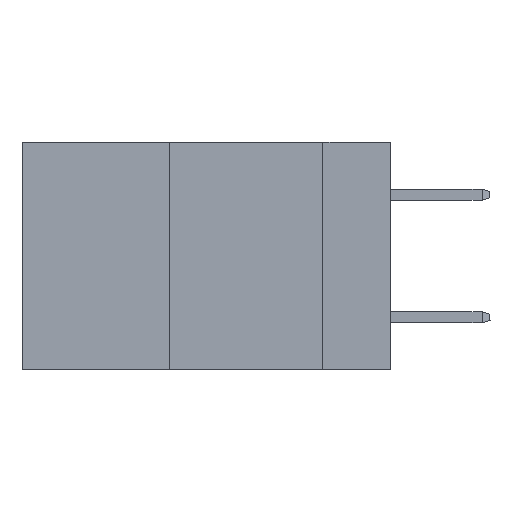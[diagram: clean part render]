
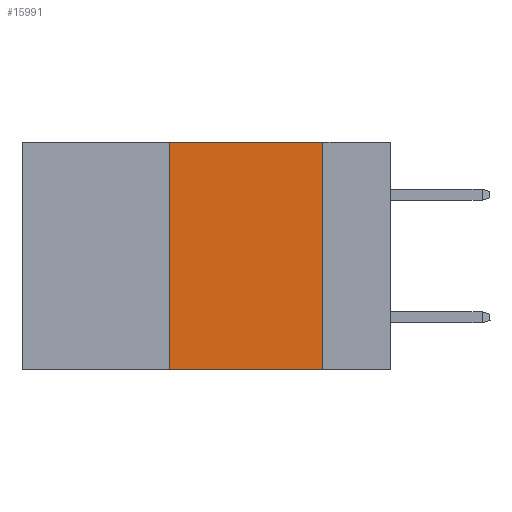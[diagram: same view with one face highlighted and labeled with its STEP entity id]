
A CAD part, left-side view. The second image highlights one B-rep face of the part: STEP entity #15991.
In plain terms, the highlighted planar face has unit normal (-1, 0, 0).
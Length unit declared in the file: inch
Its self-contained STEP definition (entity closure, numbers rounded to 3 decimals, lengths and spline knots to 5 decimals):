
#643 = CARTESIAN_POINT ( 'NONE',  ( 0., 0.6, 0. ) ) ;
#4581 = VERTEX_POINT ( 'NONE', #21005 ) ;
#7000 = EDGE_CURVE ( 'NONE', #4581, #27219, #23626, .T. ) ;
#7604 = EDGE_CURVE ( 'NONE', #27219, #26517, #26602, .T. ) ;
#8056 = AXIS2_PLACEMENT_3D ( 'NONE', #12848, #10440, #13199 ) ;
#8575 = DIRECTION ( 'NONE',  ( 0., 0., -1. ) ) ;
#10440 = DIRECTION ( 'NONE',  ( 1., 0., 0. ) ) ;
#10916 = CARTESIAN_POINT ( 'NONE',  ( 0., 0.6, -0.37 ) ) ;
#11458 = DIRECTION ( 'NONE',  ( 0., -1., 0. ) ) ;
#11513 = EDGE_LOOP ( 'NONE', ( #23986, #29584, #23904, #30124 ) ) ;
#12848 = CARTESIAN_POINT ( 'NONE',  ( 0., 0.6, 0. ) ) ;
#13199 = DIRECTION ( 'NONE',  ( 0., 0., -1. ) ) ;
#15375 = EDGE_CURVE ( 'NONE', #35137, #4581, #23863, .T. ) ;
#15991 = ADVANCED_FACE ( 'NONE', ( #25565 ), #26782, .F. ) ;
#16238 = VECTOR ( 'NONE', #19378, 39.37008 ) ;
#17116 = VECTOR ( 'NONE', #11458, 39.37008 ) ;
#19378 = DIRECTION ( 'NONE',  ( 0., -1., 0. ) ) ;
#20238 = CARTESIAN_POINT ( 'NONE',  ( 0., 0.11, -0.37 ) ) ;
#21005 = CARTESIAN_POINT ( 'NONE',  ( 0., 0.36, 0. ) ) ;
#21070 = CARTESIAN_POINT ( 'NONE',  ( 0., 0.36, 0. ) ) ;
#22234 = EDGE_CURVE ( 'NONE', #35137, #26517, #23641, .T. ) ;
#22790 = CARTESIAN_POINT ( 'NONE',  ( 0., 0.36, -0.37 ) ) ;
#23626 = LINE ( 'NONE', #643, #17116 ) ;
#23641 = LINE ( 'NONE', #10916, #16238 ) ;
#23858 = DIRECTION ( 'NONE',  ( 0., 0., 1. ) ) ;
#23863 = LINE ( 'NONE', #21070, #35088 ) ;
#23904 = ORIENTED_EDGE ( 'NONE', *, *, #15375, .F. ) ;
#23986 = ORIENTED_EDGE ( 'NONE', *, *, #7604, .F. ) ;
#24905 = CARTESIAN_POINT ( 'NONE',  ( 0., 0.11, 0. ) ) ;
#25565 = FACE_OUTER_BOUND ( 'NONE', #11513, .T. ) ;
#25589 = CARTESIAN_POINT ( 'NONE',  ( 0., 0.11, 0. ) ) ;
#26517 = VERTEX_POINT ( 'NONE', #20238 ) ;
#26602 = LINE ( 'NONE', #24905, #27023 ) ;
#26782 = PLANE ( 'NONE',  #8056 ) ;
#27023 = VECTOR ( 'NONE', #8575, 39.37008 ) ;
#27219 = VERTEX_POINT ( 'NONE', #25589 ) ;
#29584 = ORIENTED_EDGE ( 'NONE', *, *, #7000, .F. ) ;
#30124 = ORIENTED_EDGE ( 'NONE', *, *, #22234, .T. ) ;
#35088 = VECTOR ( 'NONE', #23858, 39.37008 ) ;
#35137 = VERTEX_POINT ( 'NONE', #22790 ) ;
